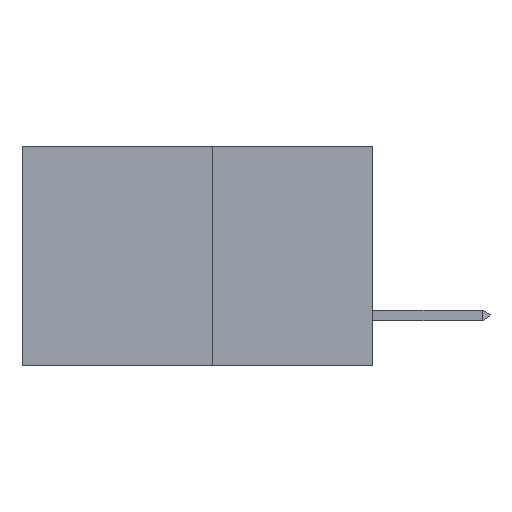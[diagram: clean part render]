
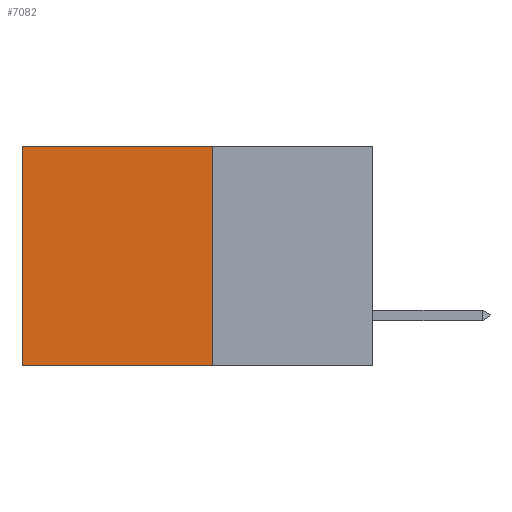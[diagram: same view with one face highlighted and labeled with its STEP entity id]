
A CAD part, left-side view. The second image highlights one B-rep face of the part: STEP entity #7082.
In plain terms, the highlighted planar face has unit normal (-1, 0, 0).
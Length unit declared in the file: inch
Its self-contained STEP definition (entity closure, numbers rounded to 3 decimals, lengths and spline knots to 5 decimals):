
#1039 = VERTEX_POINT ( 'NONE', #5886 ) ;
#1447 = VECTOR ( 'NONE', #20035, 39.37008 ) ;
#3007 = VERTEX_POINT ( 'NONE', #12638 ) ;
#4709 = CARTESIAN_POINT ( 'NONE',  ( 0.277, 0.59, -0.37 ) ) ;
#4789 = LINE ( 'NONE', #12436, #18894 ) ;
#4983 = CARTESIAN_POINT ( 'NONE',  ( 0.277, 0.59, 0. ) ) ;
#5886 = CARTESIAN_POINT ( 'NONE',  ( 0.277, 0.59, -0.37 ) ) ;
#6779 = AXIS2_PLACEMENT_3D ( 'NONE', #21102, #21082, #21029 ) ;
#7048 = DIRECTION ( 'NONE',  ( 0., 1., 0. ) ) ;
#7082 = ADVANCED_FACE ( 'NONE', ( #15405 ), #21224, .F. ) ;
#7626 = VECTOR ( 'NONE', #12034, 39.37008 ) ;
#8097 = EDGE_CURVE ( 'NONE', #12240, #1039, #21762, .T. ) ;
#11228 = ORIENTED_EDGE ( 'NONE', *, *, #22542, .T. ) ;
#11284 = LINE ( 'NONE', #18125, #1447 ) ;
#12034 = DIRECTION ( 'NONE',  ( 0., 0., -1. ) ) ;
#12240 = VERTEX_POINT ( 'NONE', #4983 ) ;
#12436 = CARTESIAN_POINT ( 'NONE',  ( 0.277, 0.27, 0. ) ) ;
#12638 = CARTESIAN_POINT ( 'NONE',  ( 0.277, 0.27, -0.37 ) ) ;
#13201 = ORIENTED_EDGE ( 'NONE', *, *, #22586, .F. ) ;
#13754 = ORIENTED_EDGE ( 'NONE', *, *, #8097, .T. ) ;
#15405 = FACE_OUTER_BOUND ( 'NONE', #23235, .T. ) ;
#15449 = EDGE_CURVE ( 'NONE', #20454, #3007, #11284, .T. ) ;
#17177 = ORIENTED_EDGE ( 'NONE', *, *, #15449, .F. ) ;
#17696 = VECTOR ( 'NONE', #7048, 39.37008 ) ;
#18125 = CARTESIAN_POINT ( 'NONE',  ( 0.277, 0.27, -0.37 ) ) ;
#18894 = VECTOR ( 'NONE', #19770, 39.37008 ) ;
#19770 = DIRECTION ( 'NONE',  ( 0., 1., 0. ) ) ;
#20035 = DIRECTION ( 'NONE',  ( 0., 0., -1. ) ) ;
#20454 = VERTEX_POINT ( 'NONE', #21094 ) ;
#21029 = DIRECTION ( 'NONE',  ( 0., 0., -1. ) ) ;
#21082 = DIRECTION ( 'NONE',  ( 1., 0., 0. ) ) ;
#21094 = CARTESIAN_POINT ( 'NONE',  ( 0.277, 0.27, 0. ) ) ;
#21102 = CARTESIAN_POINT ( 'NONE',  ( 0.277, 0.27, -0.37 ) ) ;
#21224 = PLANE ( 'NONE',  #6779 ) ;
#21762 = LINE ( 'NONE', #4709, #7626 ) ;
#22542 = EDGE_CURVE ( 'NONE', #20454, #12240, #4789, .T. ) ;
#22586 = EDGE_CURVE ( 'NONE', #3007, #1039, #22662, .T. ) ;
#22662 = LINE ( 'NONE', #23530, #17696 ) ;
#23235 = EDGE_LOOP ( 'NONE', ( #13754, #13201, #17177, #11228 ) ) ;
#23530 = CARTESIAN_POINT ( 'NONE',  ( 0.277, 0.27, -0.37 ) ) ;
